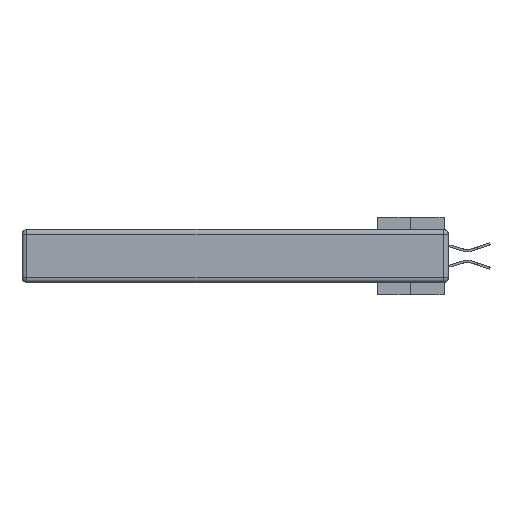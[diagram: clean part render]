
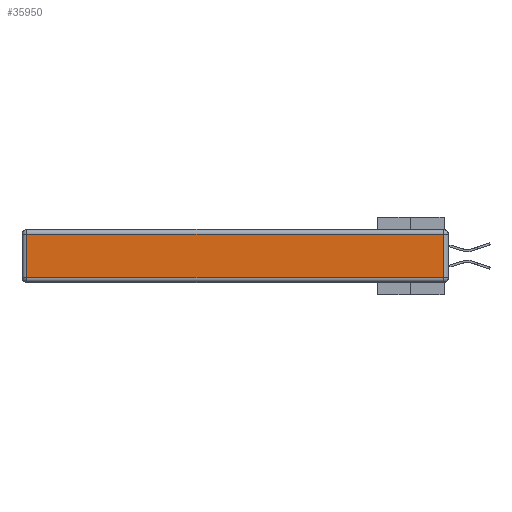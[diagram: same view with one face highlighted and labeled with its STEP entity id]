
A CAD part, left-side view. The second image highlights one B-rep face of the part: STEP entity #35950.
In plain terms, the highlighted planar face has unit normal (-1, 0, 0).
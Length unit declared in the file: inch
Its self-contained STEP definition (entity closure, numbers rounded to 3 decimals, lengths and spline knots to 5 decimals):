
#187 = ORIENTED_EDGE ( 'NONE', *, *, #16453, .T. ) ;
#1469 = EDGE_LOOP ( 'NONE', ( #31541, #34146, #20900, #187 ) ) ;
#3900 = CARTESIAN_POINT ( 'NONE',  ( 0., 2.72, -0.03 ) ) ;
#4063 = CARTESIAN_POINT ( 'NONE',  ( 0., 2.72, -0.343 ) ) ;
#4197 = DIRECTION ( 'NONE',  ( 0., 0., 1. ) ) ;
#4556 = LINE ( 'NONE', #20612, #33241 ) ;
#9676 = FACE_OUTER_BOUND ( 'NONE', #1469, .T. ) ;
#9756 = DIRECTION ( 'NONE',  ( 0., 0., 1. ) ) ;
#10011 = CARTESIAN_POINT ( 'NONE',  ( 0., 0.03, -0.343 ) ) ;
#10180 = DIRECTION ( 'NONE',  ( -1., 0., 0. ) ) ;
#13313 = LINE ( 'NONE', #10011, #16553 ) ;
#13757 = LINE ( 'NONE', #4063, #35465 ) ;
#14156 = LINE ( 'NONE', #32621, #15101 ) ;
#14612 = CARTESIAN_POINT ( 'NONE',  ( 0., 0.03, -0.03 ) ) ;
#14646 = CARTESIAN_POINT ( 'NONE',  ( 0., 0.03, -0.313 ) ) ;
#15101 = VECTOR ( 'NONE', #29292, 39.37008 ) ;
#16413 = PLANE ( 'NONE',  #27595 ) ;
#16453 = EDGE_CURVE ( 'NONE', #29322, #33793, #13757, .T. ) ;
#16553 = VECTOR ( 'NONE', #9756, 39.37008 ) ;
#16963 = CARTESIAN_POINT ( 'NONE',  ( 0., 2.72, -0.313 ) ) ;
#20612 = CARTESIAN_POINT ( 'NONE',  ( 0., 2.75, -0.03 ) ) ;
#20900 = ORIENTED_EDGE ( 'NONE', *, *, #30304, .T. ) ;
#22019 = EDGE_CURVE ( 'NONE', #33967, #34354, #13313, .T. ) ;
#22666 = EDGE_CURVE ( 'NONE', #33793, #33967, #14156, .T. ) ;
#27595 = AXIS2_PLACEMENT_3D ( 'NONE', #33692, #10180, #4197 ) ;
#29292 = DIRECTION ( 'NONE',  ( 0., -1., 0. ) ) ;
#29322 = VERTEX_POINT ( 'NONE', #3900 ) ;
#30304 = EDGE_CURVE ( 'NONE', #34354, #29322, #4556, .T. ) ;
#31541 = ORIENTED_EDGE ( 'NONE', *, *, #22666, .T. ) ;
#32621 = CARTESIAN_POINT ( 'NONE',  ( 0., 0., -0.313 ) ) ;
#33241 = VECTOR ( 'NONE', #35202, 39.37008 ) ;
#33692 = CARTESIAN_POINT ( 'NONE',  ( 0., 0., -0.343 ) ) ;
#33793 = VERTEX_POINT ( 'NONE', #16963 ) ;
#33811 = DIRECTION ( 'NONE',  ( 0., 0., -1. ) ) ;
#33967 = VERTEX_POINT ( 'NONE', #14646 ) ;
#34146 = ORIENTED_EDGE ( 'NONE', *, *, #22019, .T. ) ;
#34354 = VERTEX_POINT ( 'NONE', #14612 ) ;
#35202 = DIRECTION ( 'NONE',  ( 0., 1., 0. ) ) ;
#35465 = VECTOR ( 'NONE', #33811, 39.37008 ) ;
#35950 = ADVANCED_FACE ( 'NONE', ( #9676 ), #16413, .T. ) ;
